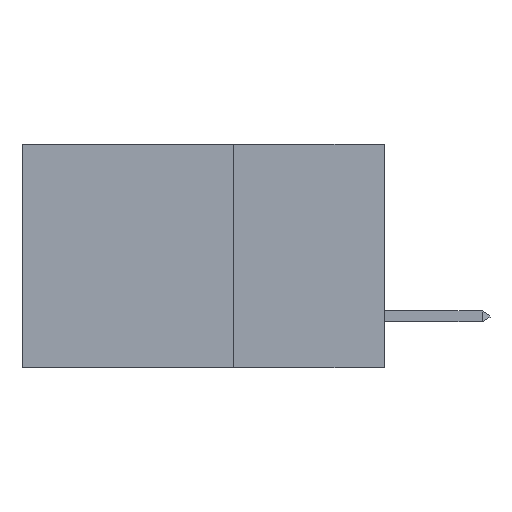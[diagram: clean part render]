
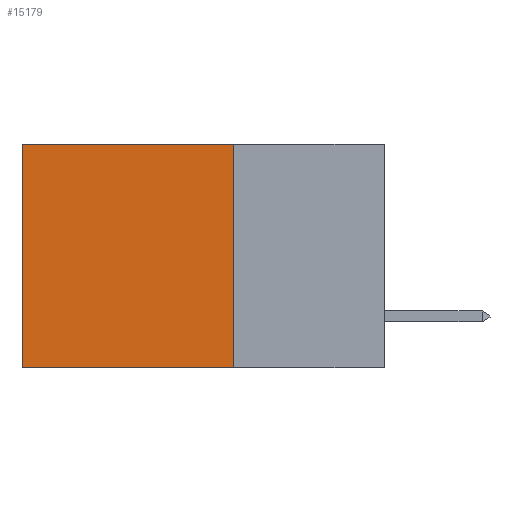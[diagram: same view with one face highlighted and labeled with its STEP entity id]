
A CAD part, left-side view. The second image highlights one B-rep face of the part: STEP entity #15179.
In plain terms, the highlighted planar face has unit normal (-1, 0, 0).
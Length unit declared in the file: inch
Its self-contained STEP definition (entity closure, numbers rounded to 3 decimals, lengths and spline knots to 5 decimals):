
#148 = DIRECTION ( 'NONE',  ( 0., 0., -1. ) ) ;
#828 = DIRECTION ( 'NONE',  ( 0., 0., -1. ) ) ;
#1206 = FACE_OUTER_BOUND ( 'NONE', #8101, .T. ) ;
#1239 = ORIENTED_EDGE ( 'NONE', *, *, #13556, .T. ) ;
#1860 = ORIENTED_EDGE ( 'NONE', *, *, #6083, .F. ) ;
#2399 = VERTEX_POINT ( 'NONE', #16791 ) ;
#2466 = CARTESIAN_POINT ( 'NONE',  ( 0.2875, 0.25, -0.37 ) ) ;
#3072 = VECTOR ( 'NONE', #11479, 39.37008 ) ;
#3382 = ORIENTED_EDGE ( 'NONE', *, *, #4812, .F. ) ;
#3541 = LINE ( 'NONE', #11585, #11046 ) ;
#4009 = VECTOR ( 'NONE', #148, 39.37008 ) ;
#4036 = DIRECTION ( 'NONE',  ( 0., 1., 0. ) ) ;
#4812 = EDGE_CURVE ( 'NONE', #2399, #8865, #10614, .T. ) ;
#4829 = VERTEX_POINT ( 'NONE', #18780 ) ;
#5015 = VERTEX_POINT ( 'NONE', #16270 ) ;
#6083 = EDGE_CURVE ( 'NONE', #5015, #2399, #15573, .T. ) ;
#6111 = CARTESIAN_POINT ( 'NONE',  ( 0.2875, 0.25, 0. ) ) ;
#6370 = CARTESIAN_POINT ( 'NONE',  ( 0.2875, 0.6, 0. ) ) ;
#7646 = DIRECTION ( 'NONE',  ( 0., 0., -1. ) ) ;
#8096 = LINE ( 'NONE', #6370, #4009 ) ;
#8101 = EDGE_LOOP ( 'NONE', ( #1239, #3382, #1860, #14493 ) ) ;
#8548 = CARTESIAN_POINT ( 'NONE',  ( 0.2875, 0.25, 0. ) ) ;
#8865 = VERTEX_POINT ( 'NONE', #12450 ) ;
#10614 = LINE ( 'NONE', #2466, #3072 ) ;
#11046 = VECTOR ( 'NONE', #4036, 39.37008 ) ;
#11479 = DIRECTION ( 'NONE',  ( 0., 1., 0. ) ) ;
#11585 = CARTESIAN_POINT ( 'NONE',  ( 0.2875, 0.25, 0. ) ) ;
#12156 = VECTOR ( 'NONE', #828, 39.37008 ) ;
#12450 = CARTESIAN_POINT ( 'NONE',  ( 0.2875, 0.6, -0.37 ) ) ;
#13279 = EDGE_CURVE ( 'NONE', #5015, #4829, #3541, .T. ) ;
#13424 = PLANE ( 'NONE',  #18493 ) ;
#13556 = EDGE_CURVE ( 'NONE', #4829, #8865, #8096, .T. ) ;
#14493 = ORIENTED_EDGE ( 'NONE', *, *, #13279, .T. ) ;
#15179 = ADVANCED_FACE ( 'NONE', ( #1206 ), #13424, .F. ) ;
#15573 = LINE ( 'NONE', #8548, #12156 ) ;
#16270 = CARTESIAN_POINT ( 'NONE',  ( 0.2875, 0.25, 0. ) ) ;
#16313 = DIRECTION ( 'NONE',  ( 1., 0., 0. ) ) ;
#16791 = CARTESIAN_POINT ( 'NONE',  ( 0.2875, 0.25, -0.37 ) ) ;
#18493 = AXIS2_PLACEMENT_3D ( 'NONE', #6111, #16313, #7646 ) ;
#18780 = CARTESIAN_POINT ( 'NONE',  ( 0.2875, 0.6, 0. ) ) ;
